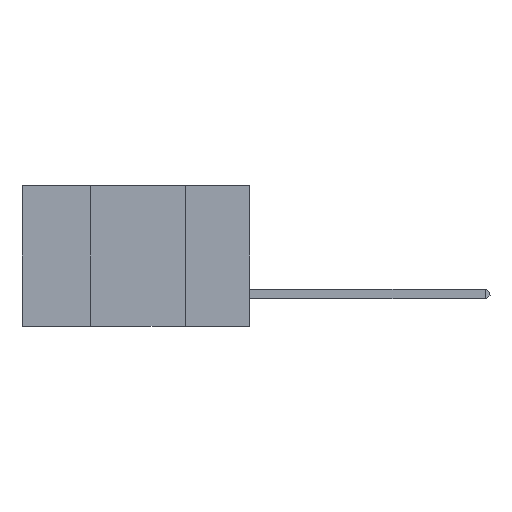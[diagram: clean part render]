
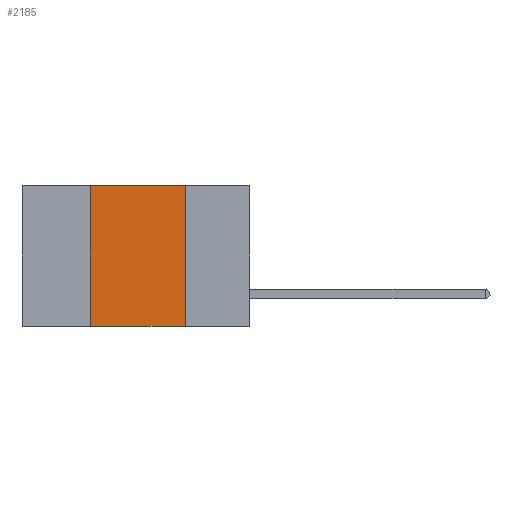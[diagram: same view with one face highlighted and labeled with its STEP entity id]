
A CAD part, left-side view. The second image highlights one B-rep face of the part: STEP entity #2185.
In plain terms, the highlighted planar face has unit normal (-1, 0, 0).
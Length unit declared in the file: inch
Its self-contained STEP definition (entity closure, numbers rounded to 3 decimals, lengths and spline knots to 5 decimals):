
#211 = DIRECTION ( 'NONE',  ( 1., 0., 0. ) ) ;
#282 = ORIENTED_EDGE ( 'NONE', *, *, #13989, .T. ) ;
#964 = VECTOR ( 'NONE', #4301, 39.37008 ) ;
#2185 = ADVANCED_FACE ( 'NONE', ( #10470 ), #5386, .F. ) ;
#2647 = CARTESIAN_POINT ( 'NONE',  ( 0., 0.42, -0.37 ) ) ;
#3282 = LINE ( 'NONE', #15731, #9404 ) ;
#3643 = AXIS2_PLACEMENT_3D ( 'NONE', #13355, #211, #7908 ) ;
#3754 = VERTEX_POINT ( 'NONE', #11391 ) ;
#3808 = EDGE_CURVE ( 'NONE', #9708, #16009, #9517, .T. ) ;
#4195 = VECTOR ( 'NONE', #10263, 39.37008 ) ;
#4301 = DIRECTION ( 'NONE',  ( 0., 0., 1. ) ) ;
#4719 = DIRECTION ( 'NONE',  ( 0., -1., 0. ) ) ;
#4845 = EDGE_LOOP ( 'NONE', ( #6065, #12241, #5093, #282 ) ) ;
#5093 = ORIENTED_EDGE ( 'NONE', *, *, #16126, .F. ) ;
#5125 = VECTOR ( 'NONE', #4719, 39.37008 ) ;
#5386 = PLANE ( 'NONE',  #3643 ) ;
#5817 = CARTESIAN_POINT ( 'NONE',  ( 0., 0.42, 0. ) ) ;
#6065 = ORIENTED_EDGE ( 'NONE', *, *, #7641, .F. ) ;
#7641 = EDGE_CURVE ( 'NONE', #16009, #3754, #3282, .T. ) ;
#7908 = DIRECTION ( 'NONE',  ( 0., 0., -1. ) ) ;
#9174 = DIRECTION ( 'NONE',  ( 0., 0., -1. ) ) ;
#9404 = VECTOR ( 'NONE', #9174, 39.37008 ) ;
#9517 = LINE ( 'NONE', #12949, #4195 ) ;
#9661 = LINE ( 'NONE', #11407, #5125 ) ;
#9708 = VERTEX_POINT ( 'NONE', #14458 ) ;
#9710 = LINE ( 'NONE', #5817, #964 ) ;
#10263 = DIRECTION ( 'NONE',  ( 0., -1., 0. ) ) ;
#10470 = FACE_OUTER_BOUND ( 'NONE', #4845, .T. ) ;
#11391 = CARTESIAN_POINT ( 'NONE',  ( 0., 0.17, -0.37 ) ) ;
#11407 = CARTESIAN_POINT ( 'NONE',  ( 0., 0.6, -0.37 ) ) ;
#12241 = ORIENTED_EDGE ( 'NONE', *, *, #3808, .F. ) ;
#12440 = VERTEX_POINT ( 'NONE', #2647 ) ;
#12949 = CARTESIAN_POINT ( 'NONE',  ( 0., 0.6, 0. ) ) ;
#13239 = CARTESIAN_POINT ( 'NONE',  ( 0., 0.17, 0. ) ) ;
#13355 = CARTESIAN_POINT ( 'NONE',  ( 0., 0.6, 0. ) ) ;
#13989 = EDGE_CURVE ( 'NONE', #12440, #3754, #9661, .T. ) ;
#14458 = CARTESIAN_POINT ( 'NONE',  ( 0., 0.42, 0. ) ) ;
#15731 = CARTESIAN_POINT ( 'NONE',  ( 0., 0.17, 0. ) ) ;
#16009 = VERTEX_POINT ( 'NONE', #13239 ) ;
#16126 = EDGE_CURVE ( 'NONE', #12440, #9708, #9710, .T. ) ;
